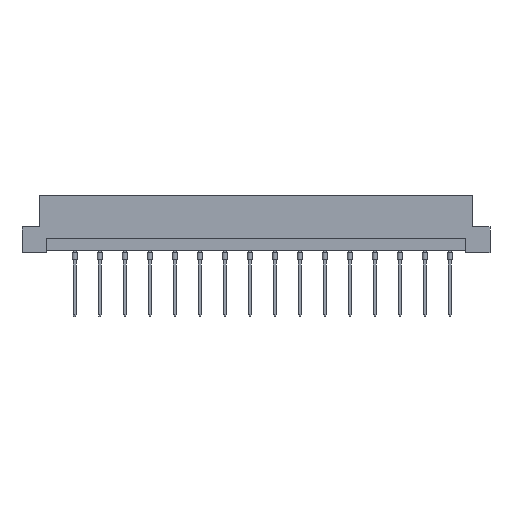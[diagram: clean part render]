
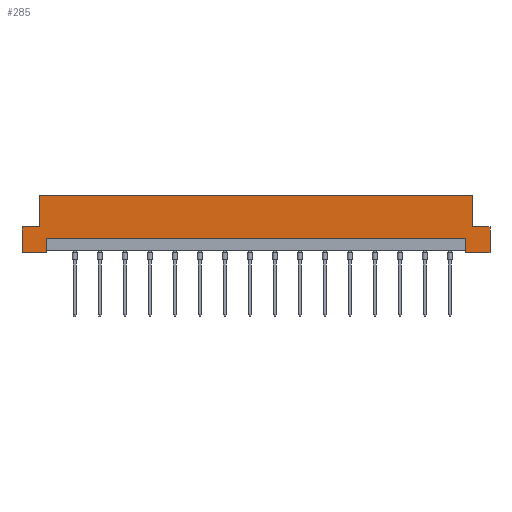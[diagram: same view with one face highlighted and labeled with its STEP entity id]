
A CAD part, front view. The second image highlights one B-rep face of the part: STEP entity #285.
In plain terms, the highlighted planar face has unit normal (0, -1, 0).
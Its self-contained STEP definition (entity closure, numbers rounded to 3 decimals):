
#212 = VERTEX_POINT ( 'NONE', #15567 ) ;
#285 = ADVANCED_FACE ( 'NONE', ( #9490 ), #2918, .F. ) ;
#518 = EDGE_CURVE ( 'NONE', #7837, #11262, #16835, .T. ) ;
#534 = CARTESIAN_POINT ( 'NONE',  ( -47.5, 0., 5.2 ) ) ;
#665 = DIRECTION ( 'NONE',  ( 0., 0., 1. ) ) ;
#954 = VECTOR ( 'NONE', #2786, 1000. ) ;
#991 = CARTESIAN_POINT ( 'NONE',  ( 42.6, 0., 2.9 ) ) ;
#1319 = CARTESIAN_POINT ( 'NONE',  ( -47.5, 0., 5.2 ) ) ;
#1330 = ORIENTED_EDGE ( 'NONE', *, *, #15859, .T. ) ;
#1457 = CARTESIAN_POINT ( 'NONE',  ( 42.6, 0., 0. ) ) ;
#1805 = VERTEX_POINT ( 'NONE', #7249 ) ;
#1836 = ORIENTED_EDGE ( 'NONE', *, *, #518, .F. ) ;
#1959 = LINE ( 'NONE', #8806, #6766 ) ;
#2034 = ORIENTED_EDGE ( 'NONE', *, *, #3097, .F. ) ;
#2586 = ORIENTED_EDGE ( 'NONE', *, *, #11455, .F. ) ;
#2679 = VECTOR ( 'NONE', #5738, 1000. ) ;
#2745 = ORIENTED_EDGE ( 'NONE', *, *, #12899, .F. ) ;
#2786 = DIRECTION ( 'NONE',  ( 0., 0., -1. ) ) ;
#2829 = DIRECTION ( 'NONE',  ( 0., 0., 1. ) ) ;
#2918 = PLANE ( 'NONE',  #12786 ) ;
#3097 = EDGE_CURVE ( 'NONE', #212, #7837, #6838, .T. ) ;
#3230 = CARTESIAN_POINT ( 'NONE',  ( -44., 0., 5.2 ) ) ;
#3347 = LINE ( 'NONE', #4914, #12329 ) ;
#3388 = ORIENTED_EDGE ( 'NONE', *, *, #10763, .F. ) ;
#3651 = CARTESIAN_POINT ( 'NONE',  ( 42.6, 0., 0.5 ) ) ;
#3679 = CARTESIAN_POINT ( 'NONE',  ( 47.5, 0., 0. ) ) ;
#3993 = EDGE_CURVE ( 'NONE', #7747, #1805, #6388, .T. ) ;
#4238 = CARTESIAN_POINT ( 'NONE',  ( -47.5, 0., 0. ) ) ;
#4285 = ORIENTED_EDGE ( 'NONE', *, *, #16632, .F. ) ;
#4393 = EDGE_CURVE ( 'NONE', #4743, #15979, #5949, .T. ) ;
#4611 = VECTOR ( 'NONE', #14403, 1000. ) ;
#4682 = VECTOR ( 'NONE', #12771, 1000. ) ;
#4743 = VERTEX_POINT ( 'NONE', #15415 ) ;
#4914 = CARTESIAN_POINT ( 'NONE',  ( 42.6, 0., 2.9 ) ) ;
#4951 = DIRECTION ( 'NONE',  ( -1., 0., 0. ) ) ;
#4974 = CARTESIAN_POINT ( 'NONE',  ( -47.5, 0., 0. ) ) ;
#4989 = CARTESIAN_POINT ( 'NONE',  ( 44., 0., 5.2 ) ) ;
#5114 = ORIENTED_EDGE ( 'NONE', *, *, #16787, .F. ) ;
#5124 = DIRECTION ( 'NONE',  ( 0., 0., -1. ) ) ;
#5197 = ORIENTED_EDGE ( 'NONE', *, *, #4393, .F. ) ;
#5391 = VECTOR ( 'NONE', #12186, 1000. ) ;
#5738 = DIRECTION ( 'NONE',  ( 1., 0., 0. ) ) ;
#5949 = LINE ( 'NONE', #11201, #4682 ) ;
#6030 = VECTOR ( 'NONE', #4951, 1000. ) ;
#6388 = LINE ( 'NONE', #14593, #8783 ) ;
#6423 = VERTEX_POINT ( 'NONE', #7981 ) ;
#6766 = VECTOR ( 'NONE', #665, 1000. ) ;
#6838 = LINE ( 'NONE', #8468, #5391 ) ;
#7159 = VERTEX_POINT ( 'NONE', #991 ) ;
#7201 = VERTEX_POINT ( 'NONE', #3679 ) ;
#7249 = CARTESIAN_POINT ( 'NONE',  ( 47.5, 0., 5.2 ) ) ;
#7747 = VERTEX_POINT ( 'NONE', #11840 ) ;
#7829 = VERTEX_POINT ( 'NONE', #1457 ) ;
#7837 = VERTEX_POINT ( 'NONE', #4238 ) ;
#7981 = CARTESIAN_POINT ( 'NONE',  ( -42.6, 0., 2.9 ) ) ;
#8207 = VECTOR ( 'NONE', #5124, 1000. ) ;
#8468 = CARTESIAN_POINT ( 'NONE',  ( -47.5, 0., 0. ) ) ;
#8783 = VECTOR ( 'NONE', #10345, 1000. ) ;
#8806 = CARTESIAN_POINT ( 'NONE',  ( -44., 0., 5.2 ) ) ;
#9273 = LINE ( 'NONE', #13526, #954 ) ;
#9490 = FACE_OUTER_BOUND ( 'NONE', #16742, .T. ) ;
#9953 = CARTESIAN_POINT ( 'NONE',  ( -42.6, 0., 0.5 ) ) ;
#10157 = VECTOR ( 'NONE', #12471, 1000. ) ;
#10236 = DIRECTION ( 'NONE',  ( 0., 0., 1. ) ) ;
#10345 = DIRECTION ( 'NONE',  ( 1., 0., 0. ) ) ;
#10763 = EDGE_CURVE ( 'NONE', #15267, #4743, #1959, .T. ) ;
#11195 = CARTESIAN_POINT ( 'NONE',  ( -47.5, 0., 11.6 ) ) ;
#11201 = CARTESIAN_POINT ( 'NONE',  ( -47.5, 0., 11.6 ) ) ;
#11262 = VERTEX_POINT ( 'NONE', #1319 ) ;
#11455 = EDGE_CURVE ( 'NONE', #1805, #7201, #9273, .T. ) ;
#11594 = LINE ( 'NONE', #15588, #6030 ) ;
#11805 = LINE ( 'NONE', #4989, #4611 ) ;
#11840 = CARTESIAN_POINT ( 'NONE',  ( 44., 0., 5.2 ) ) ;
#12186 = DIRECTION ( 'NONE',  ( -1., 0., 0. ) ) ;
#12329 = VECTOR ( 'NONE', #13994, 1000. ) ;
#12471 = DIRECTION ( 'NONE',  ( 0., 0., -1. ) ) ;
#12771 = DIRECTION ( 'NONE',  ( 1., 0., 0. ) ) ;
#12786 = AXIS2_PLACEMENT_3D ( 'NONE', #11195, #13221, #2829 ) ;
#12834 = LINE ( 'NONE', #3651, #8207 ) ;
#12899 = EDGE_CURVE ( 'NONE', #7159, #6423, #3347, .T. ) ;
#13093 = ORIENTED_EDGE ( 'NONE', *, *, #16668, .F. ) ;
#13221 = DIRECTION ( 'NONE',  ( 0., 1., 0. ) ) ;
#13526 = CARTESIAN_POINT ( 'NONE',  ( 47.5, 0., 0. ) ) ;
#13605 = VECTOR ( 'NONE', #10236, 1000. ) ;
#13994 = DIRECTION ( 'NONE',  ( -1., 0., 0. ) ) ;
#14023 = EDGE_CURVE ( 'NONE', #7159, #7829, #12834, .T. ) ;
#14031 = LINE ( 'NONE', #534, #2679 ) ;
#14323 = CARTESIAN_POINT ( 'NONE',  ( 44., 0., 11.6 ) ) ;
#14403 = DIRECTION ( 'NONE',  ( 0., 0., 1. ) ) ;
#14557 = ORIENTED_EDGE ( 'NONE', *, *, #3993, .F. ) ;
#14593 = CARTESIAN_POINT ( 'NONE',  ( 47.5, 0., 5.2 ) ) ;
#15267 = VERTEX_POINT ( 'NONE', #3230 ) ;
#15415 = CARTESIAN_POINT ( 'NONE',  ( -44., 0., 11.6 ) ) ;
#15567 = CARTESIAN_POINT ( 'NONE',  ( -42.6, 0., 0. ) ) ;
#15588 = CARTESIAN_POINT ( 'NONE',  ( -47.5, 0., 0. ) ) ;
#15859 = EDGE_CURVE ( 'NONE', #7747, #15979, #11805, .T. ) ;
#15979 = VERTEX_POINT ( 'NONE', #14323 ) ;
#16472 = LINE ( 'NONE', #9953, #10157 ) ;
#16477 = ORIENTED_EDGE ( 'NONE', *, *, #14023, .T. ) ;
#16632 = EDGE_CURVE ( 'NONE', #6423, #212, #16472, .T. ) ;
#16668 = EDGE_CURVE ( 'NONE', #11262, #15267, #14031, .T. ) ;
#16742 = EDGE_LOOP ( 'NONE', ( #2745, #16477, #5114, #2586, #14557, #1330, #5197, #3388, #13093, #1836, #2034, #4285 ) ) ;
#16787 = EDGE_CURVE ( 'NONE', #7201, #7829, #11594, .T. ) ;
#16835 = LINE ( 'NONE', #4974, #13605 ) ;
